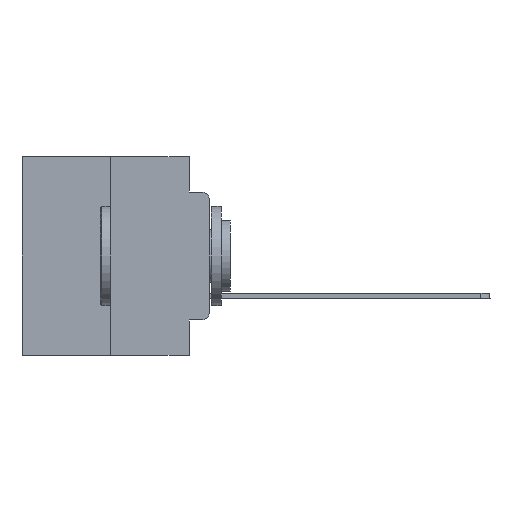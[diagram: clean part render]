
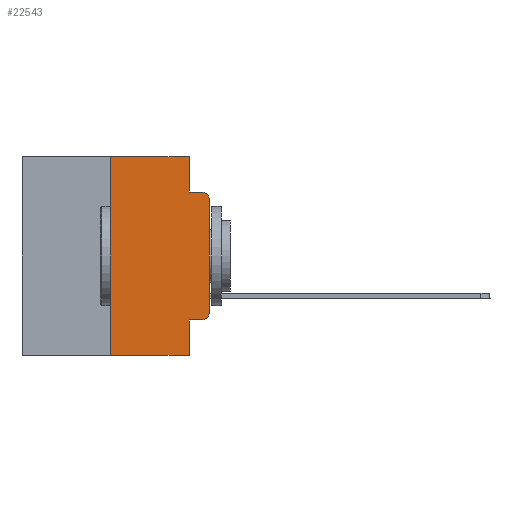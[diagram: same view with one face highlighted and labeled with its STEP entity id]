
A CAD part, left-side view. The second image highlights one B-rep face of the part: STEP entity #22543.
In plain terms, the highlighted planar face has unit normal (-1, 0, 0).
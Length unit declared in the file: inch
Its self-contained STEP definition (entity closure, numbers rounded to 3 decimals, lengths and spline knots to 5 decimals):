
#274 = CIRCLE ( 'NONE', #5358, 0.02 ) ;
#428 = VERTEX_POINT ( 'NONE', #16422 ) ;
#943 = DIRECTION ( 'NONE',  ( 0., -1., 0. ) ) ;
#1046 = CARTESIAN_POINT ( 'NONE',  ( 0., 0.473, 0. ) ) ;
#1371 = ORIENTED_EDGE ( 'NONE', *, *, #4549, .T. ) ;
#1423 = ORIENTED_EDGE ( 'NONE', *, *, #20840, .T. ) ;
#2015 = LINE ( 'NONE', #1046, #2683 ) ;
#2264 = LINE ( 'NONE', #20490, #27850 ) ;
#2269 = EDGE_CURVE ( 'NONE', #12920, #12641, #2015, .T. ) ;
#2504 = CIRCLE ( 'NONE', #18714, 0.02 ) ;
#2628 = EDGE_CURVE ( 'NONE', #27955, #6037, #274, .T. ) ;
#2683 = VECTOR ( 'NONE', #7714, 39.37008 ) ;
#3373 = VERTEX_POINT ( 'NONE', #12393 ) ;
#3923 = DIRECTION ( 'NONE',  ( 0., -1., 0. ) ) ;
#4259 = ORIENTED_EDGE ( 'NONE', *, *, #2628, .T. ) ;
#4549 = EDGE_CURVE ( 'NONE', #3373, #428, #26455, .T. ) ;
#4867 = CARTESIAN_POINT ( 'NONE',  ( 0., 0.051, -0.4115 ) ) ;
#5041 = CARTESIAN_POINT ( 'NONE',  ( 0., 0.051, -0.0885 ) ) ;
#5170 = ORIENTED_EDGE ( 'NONE', *, *, #20924, .T. ) ;
#5226 = CARTESIAN_POINT ( 'NONE',  ( 0., 0.02, -0.1085 ) ) ;
#5358 = AXIS2_PLACEMENT_3D ( 'NONE', #5226, #26701, #13768 ) ;
#5994 = FACE_OUTER_BOUND ( 'NONE', #13043, .T. ) ;
#6037 = VERTEX_POINT ( 'NONE', #17388 ) ;
#7078 = CARTESIAN_POINT ( 'NONE',  ( 0., 0.02, -0.3915 ) ) ;
#7714 = DIRECTION ( 'NONE',  ( 0., -1., 0. ) ) ;
#7764 = EDGE_CURVE ( 'NONE', #14682, #12920, #27871, .T. ) ;
#8684 = LINE ( 'NONE', #22614, #22028 ) ;
#8743 = EDGE_CURVE ( 'NONE', #3373, #23248, #2264, .T. ) ;
#9195 = DIRECTION ( 'NONE',  ( -1., 0., 0. ) ) ;
#9550 = DIRECTION ( 'NONE',  ( 1., 0., 0. ) ) ;
#9813 = CARTESIAN_POINT ( 'NONE',  ( 0., 0., 0. ) ) ;
#9911 = LINE ( 'NONE', #5041, #17797 ) ;
#9957 = EDGE_CURVE ( 'NONE', #25295, #27955, #15183, .T. ) ;
#10022 = EDGE_CURVE ( 'NONE', #12641, #26611, #8684, .T. ) ;
#10035 = CARTESIAN_POINT ( 'NONE',  ( 0., 0.473, -0.5 ) ) ;
#10758 = CARTESIAN_POINT ( 'NONE',  ( 0., 0.051, 0. ) ) ;
#11312 = ORIENTED_EDGE ( 'NONE', *, *, #2269, .F. ) ;
#12393 = CARTESIAN_POINT ( 'NONE',  ( 0., 0.051, -0.4115 ) ) ;
#12641 = VERTEX_POINT ( 'NONE', #10758 ) ;
#12818 = CARTESIAN_POINT ( 'NONE',  ( 0., 0.051, -0.0885 ) ) ;
#12883 = ORIENTED_EDGE ( 'NONE', *, *, #8743, .F. ) ;
#12920 = VERTEX_POINT ( 'NONE', #14222 ) ;
#12939 = CARTESIAN_POINT ( 'NONE',  ( 0., 0., -0.1085 ) ) ;
#13043 = EDGE_LOOP ( 'NONE', ( #14722, #4259, #22866, #18857, #11312, #16637, #5170, #12883, #1371, #1423 ) ) ;
#13768 = DIRECTION ( 'NONE',  ( 0., 0., -1. ) ) ;
#14222 = CARTESIAN_POINT ( 'NONE',  ( 0., 0.25, 0. ) ) ;
#14321 = VECTOR ( 'NONE', #943, 39.37008 ) ;
#14350 = PLANE ( 'NONE',  #16909 ) ;
#14396 = DIRECTION ( 'NONE',  ( 0., -1., 0. ) ) ;
#14682 = VERTEX_POINT ( 'NONE', #22931 ) ;
#14722 = ORIENTED_EDGE ( 'NONE', *, *, #9957, .T. ) ;
#15183 = LINE ( 'NONE', #9813, #23384 ) ;
#15960 = CARTESIAN_POINT ( 'NONE',  ( 0., 0.051, -0.5 ) ) ;
#16293 = VECTOR ( 'NONE', #17650, 39.37008 ) ;
#16369 = EDGE_CURVE ( 'NONE', #26611, #6037, #9911, .T. ) ;
#16422 = CARTESIAN_POINT ( 'NONE',  ( 0., 0.02, -0.4115 ) ) ;
#16564 = CARTESIAN_POINT ( 'NONE',  ( 0., 0.473, 0. ) ) ;
#16637 = ORIENTED_EDGE ( 'NONE', *, *, #7764, .F. ) ;
#16909 = AXIS2_PLACEMENT_3D ( 'NONE', #16564, #9550, #24815 ) ;
#17358 = CARTESIAN_POINT ( 'NONE',  ( 0., 0., -0.3915 ) ) ;
#17388 = CARTESIAN_POINT ( 'NONE',  ( 0., 0.02, -0.0885 ) ) ;
#17650 = DIRECTION ( 'NONE',  ( 0., 0., 1. ) ) ;
#17797 = VECTOR ( 'NONE', #3923, 39.37008 ) ;
#18714 = AXIS2_PLACEMENT_3D ( 'NONE', #7078, #9195, #24478 ) ;
#18857 = ORIENTED_EDGE ( 'NONE', *, *, #10022, .F. ) ;
#20068 = VECTOR ( 'NONE', #14396, 39.37008 ) ;
#20490 = CARTESIAN_POINT ( 'NONE',  ( 0., 0.051, 0. ) ) ;
#20840 = EDGE_CURVE ( 'NONE', #428, #25295, #2504, .T. ) ;
#20855 = LINE ( 'NONE', #10035, #14321 ) ;
#20924 = EDGE_CURVE ( 'NONE', #14682, #23248, #20855, .T. ) ;
#22028 = VECTOR ( 'NONE', #24785, 39.37008 ) ;
#22543 = ADVANCED_FACE ( 'NONE', ( #5994 ), #14350, .F. ) ;
#22614 = CARTESIAN_POINT ( 'NONE',  ( 0., 0.051, 0. ) ) ;
#22866 = ORIENTED_EDGE ( 'NONE', *, *, #16369, .F. ) ;
#22931 = CARTESIAN_POINT ( 'NONE',  ( 0., 0.25, -0.5 ) ) ;
#23248 = VERTEX_POINT ( 'NONE', #15960 ) ;
#23384 = VECTOR ( 'NONE', #27064, 39.37008 ) ;
#24478 = DIRECTION ( 'NONE',  ( 0., 0., -1. ) ) ;
#24785 = DIRECTION ( 'NONE',  ( 0., 0., -1. ) ) ;
#24815 = DIRECTION ( 'NONE',  ( 0., 0., -1. ) ) ;
#24816 = DIRECTION ( 'NONE',  ( 0., 0., -1. ) ) ;
#25295 = VERTEX_POINT ( 'NONE', #17358 ) ;
#26402 = CARTESIAN_POINT ( 'NONE',  ( 0., 0.25, 0. ) ) ;
#26455 = LINE ( 'NONE', #4867, #20068 ) ;
#26611 = VERTEX_POINT ( 'NONE', #12818 ) ;
#26701 = DIRECTION ( 'NONE',  ( -1., 0., 0. ) ) ;
#27064 = DIRECTION ( 'NONE',  ( 0., 0., 1. ) ) ;
#27850 = VECTOR ( 'NONE', #24816, 39.37008 ) ;
#27871 = LINE ( 'NONE', #26402, #16293 ) ;
#27955 = VERTEX_POINT ( 'NONE', #12939 ) ;
